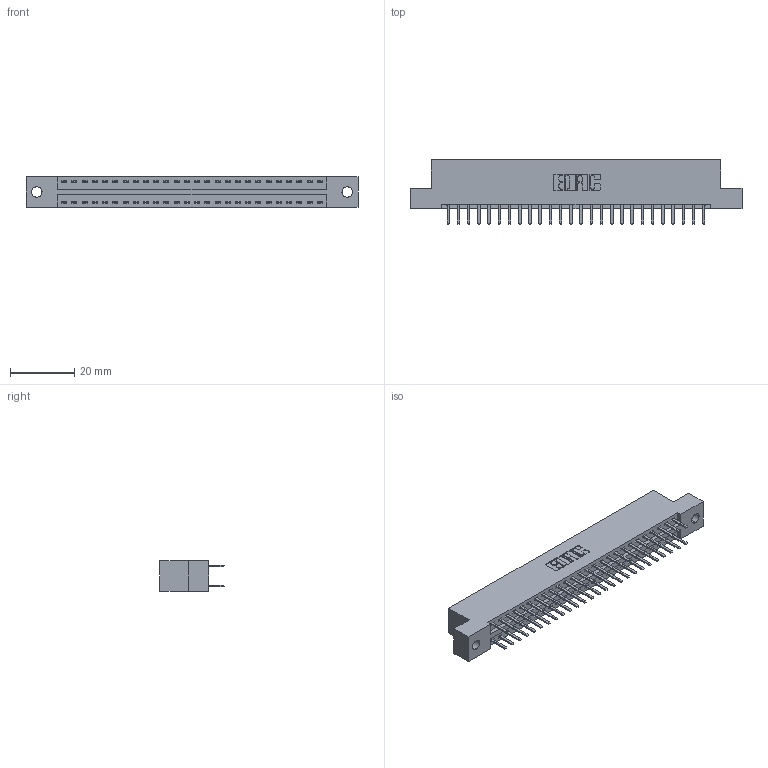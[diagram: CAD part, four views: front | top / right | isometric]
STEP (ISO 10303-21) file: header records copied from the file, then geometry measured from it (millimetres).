
FILE_DESCRIPTION (( 'STEP AP203' ), '1' );
FILE_NAME ('346-052-520-202.STEP', '2018-08-27T23:28:10', ( '' ), ( '' ), 'SwSTEP 2.0', 'SolidWorks 2016', '' );
FILE_SCHEMA (( 'CONFIG_CONTROL_DESIGN' ));
Length unit declared in the file: inch
Products named in the file (3): 346 Part_Flush Mounting Lugs - 0.128 Dia; 345-292-001_345-293-120; 346-052-520-202
Assembly tree (53 placements, depth 2):
  346-052-520-202
    346 Part_Flush Mounting Lugs - 0.128 Dia
    345-292-001_345-293-120  x52
Bounding box: 103.12 x 20.02 x 9.4 mm (x, y, z)
Volume: 9872.1 mm3; surface area: 12995.5 mm2
Topology: 53 solids, 53 shells, 3034 faces, 8805 edges, 5730 vertices
Faces by surface type: plane 2000, cylinder 1034
Entity records: 19239 total; most frequent: CARTESIAN_POINT 3204, ORIENTED_EDGE 3126, DIRECTION 2863, EDGE_CURVE 1563, VECTOR 1323, LINE 1323, VERTEX_POINT 1038, AXIS2_PLACEMENT_3D 770
